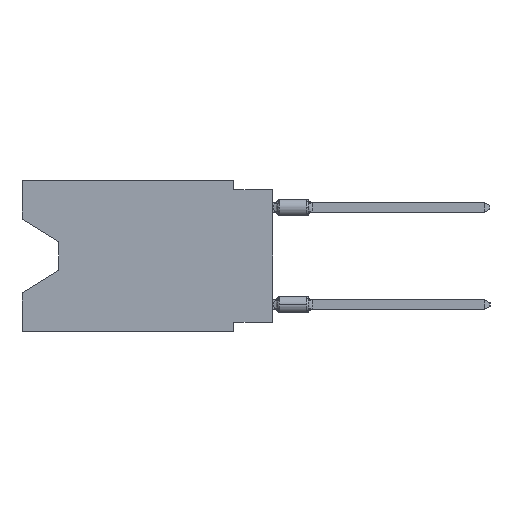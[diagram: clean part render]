
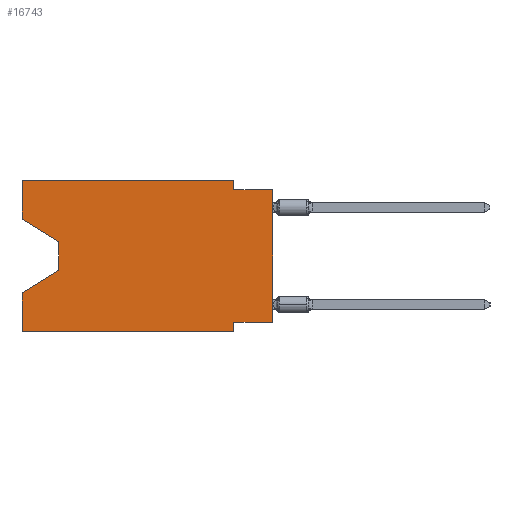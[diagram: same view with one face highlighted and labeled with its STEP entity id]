
A CAD part, left-side view. The second image highlights one B-rep face of the part: STEP entity #16743.
In plain terms, the highlighted planar face has unit normal (-1, 0, 0).
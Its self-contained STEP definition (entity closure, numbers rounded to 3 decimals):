
#596 = CARTESIAN_POINT ( 'NONE',  ( 0., 13.97, -4.013 ) ) ;
#653 = LINE ( 'NONE', #23983, #19637 ) ;
#842 = LINE ( 'NONE', #13902, #12736 ) ;
#1052 = ORIENTED_EDGE ( 'NONE', *, *, #29931, .T. ) ;
#1077 = CARTESIAN_POINT ( 'NONE',  ( 0., 2.54, -9.906 ) ) ;
#1109 = LINE ( 'NONE', #29670, #18030 ) ;
#2143 = FACE_OUTER_BOUND ( 'NONE', #13013, .T. ) ;
#2547 = DIRECTION ( 'NONE',  ( 0., -1., 0. ) ) ;
#2576 = ORIENTED_EDGE ( 'NONE', *, *, #39382, .F. ) ;
#3517 = VECTOR ( 'NONE', #20984, 1000. ) ;
#3656 = CARTESIAN_POINT ( 'NONE',  ( 0., 0., -0.635 ) ) ;
#4217 = LINE ( 'NONE', #11286, #37618 ) ;
#4833 = CARTESIAN_POINT ( 'NONE',  ( 0., 16.383, -2.546 ) ) ;
#5164 = ORIENTED_EDGE ( 'NONE', *, *, #32402, .F. ) ;
#5377 = DIRECTION ( 'NONE',  ( 0., 0., -1. ) ) ;
#6178 = VERTEX_POINT ( 'NONE', #6815 ) ;
#6801 = VERTEX_POINT ( 'NONE', #10830 ) ;
#6815 = CARTESIAN_POINT ( 'NONE',  ( 0., 2.54, -0.635 ) ) ;
#7236 = CARTESIAN_POINT ( 'NONE',  ( 0., 0., -0.635 ) ) ;
#7422 = DIRECTION ( 'NONE',  ( 0., 0., -1. ) ) ;
#7446 = VECTOR ( 'NONE', #29320, 1000. ) ;
#7562 = DIRECTION ( 'NONE',  ( 1., 0., 0. ) ) ;
#7871 = DIRECTION ( 'NONE',  ( 0., -1., 0. ) ) ;
#8173 = VERTEX_POINT ( 'NONE', #15523 ) ;
#10216 = ORIENTED_EDGE ( 'NONE', *, *, #24145, .F. ) ;
#10549 = CARTESIAN_POINT ( 'NONE',  ( 0., 2.54, 0. ) ) ;
#10830 = CARTESIAN_POINT ( 'NONE',  ( 0., 16.383, 0. ) ) ;
#11286 = CARTESIAN_POINT ( 'NONE',  ( 0., 16.383, 0. ) ) ;
#12124 = VECTOR ( 'NONE', #7871, 1000. ) ;
#12736 = VECTOR ( 'NONE', #7422, 1000. ) ;
#13013 = EDGE_LOOP ( 'NONE', ( #22837, #1052, #39787, #10216, #38677, #34655, #5164, #20052, #34958, #22917, #28257, #2576 ) ) ;
#13902 = CARTESIAN_POINT ( 'NONE',  ( 0., 13.97, -4.013 ) ) ;
#13945 = EDGE_CURVE ( 'NONE', #6801, #41479, #1109, .T. ) ;
#14997 = VECTOR ( 'NONE', #21978, 1000. ) ;
#15391 = CARTESIAN_POINT ( 'NONE',  ( 0., 16.383, -9.906 ) ) ;
#15523 = CARTESIAN_POINT ( 'NONE',  ( 0., 2.54, -9.271 ) ) ;
#15562 = LINE ( 'NONE', #31651, #14997 ) ;
#16112 = VECTOR ( 'NONE', #40861, 1000. ) ;
#16743 = ADVANCED_FACE ( 'NONE', ( #2143 ), #23850, .F. ) ;
#16860 = CARTESIAN_POINT ( 'NONE',  ( 0., 13.97, -5.893 ) ) ;
#18030 = VECTOR ( 'NONE', #22798, 1000. ) ;
#18427 = EDGE_CURVE ( 'NONE', #8173, #28318, #37100, .T. ) ;
#19011 = VECTOR ( 'NONE', #2547, 1000. ) ;
#19637 = VECTOR ( 'NONE', #39692, 1000. ) ;
#19661 = LINE ( 'NONE', #16860, #7446 ) ;
#20052 = ORIENTED_EDGE ( 'NONE', *, *, #29200, .T. ) ;
#20984 = DIRECTION ( 'NONE',  ( 0., 0., -1. ) ) ;
#21365 = CARTESIAN_POINT ( 'NONE',  ( 0., 13.97, -5.893 ) ) ;
#21547 = CARTESIAN_POINT ( 'NONE',  ( 0., 16.383, -9.906 ) ) ;
#21718 = CARTESIAN_POINT ( 'NONE',  ( 0., 16.383, -2.546 ) ) ;
#21978 = DIRECTION ( 'NONE',  ( 0., 0., -1. ) ) ;
#22300 = VERTEX_POINT ( 'NONE', #21547 ) ;
#22470 = LINE ( 'NONE', #32545, #40842 ) ;
#22726 = EDGE_CURVE ( 'NONE', #41015, #39270, #27740, .T. ) ;
#22798 = DIRECTION ( 'NONE',  ( 0., -1., 0. ) ) ;
#22837 = ORIENTED_EDGE ( 'NONE', *, *, #22726, .T. ) ;
#22917 = ORIENTED_EDGE ( 'NONE', *, *, #39469, .F. ) ;
#22973 = CARTESIAN_POINT ( 'NONE',  ( 0., 2.54, -9.906 ) ) ;
#23195 = CARTESIAN_POINT ( 'NONE',  ( 0., 16.383, 0. ) ) ;
#23850 = PLANE ( 'NONE',  #33568 ) ;
#23983 = CARTESIAN_POINT ( 'NONE',  ( 0., 0., -9.271 ) ) ;
#24145 = EDGE_CURVE ( 'NONE', #22300, #27366, #36305, .T. ) ;
#24353 = DIRECTION ( 'NONE',  ( 0., 0., 1. ) ) ;
#26185 = EDGE_CURVE ( 'NONE', #37577, #27366, #19661, .T. ) ;
#26486 = VECTOR ( 'NONE', #30275, 1000. ) ;
#27182 = LINE ( 'NONE', #7236, #12124 ) ;
#27366 = VERTEX_POINT ( 'NONE', #38624 ) ;
#27740 = LINE ( 'NONE', #21718, #16112 ) ;
#28257 = ORIENTED_EDGE ( 'NONE', *, *, #13945, .F. ) ;
#28318 = VERTEX_POINT ( 'NONE', #22973 ) ;
#29200 = EDGE_CURVE ( 'NONE', #40311, #36917, #22470, .T. ) ;
#29320 = DIRECTION ( 'NONE',  ( 0., 0.855, -0.519 ) ) ;
#29531 = DIRECTION ( 'NONE',  ( 0., 0., 1. ) ) ;
#29670 = CARTESIAN_POINT ( 'NONE',  ( 0., 16.383, 0. ) ) ;
#29931 = EDGE_CURVE ( 'NONE', #39270, #37577, #842, .T. ) ;
#30275 = DIRECTION ( 'NONE',  ( 0., 0., 1. ) ) ;
#31578 = EDGE_CURVE ( 'NONE', #22300, #28318, #41598, .T. ) ;
#31651 = CARTESIAN_POINT ( 'NONE',  ( 0., 2.54, 0. ) ) ;
#32402 = EDGE_CURVE ( 'NONE', #40311, #8173, #653, .T. ) ;
#32545 = CARTESIAN_POINT ( 'NONE',  ( 0., 0., 0. ) ) ;
#33568 = AXIS2_PLACEMENT_3D ( 'NONE', #34740, #7562, #5377 ) ;
#34086 = CARTESIAN_POINT ( 'NONE',  ( 0., 0., -9.271 ) ) ;
#34655 = ORIENTED_EDGE ( 'NONE', *, *, #18427, .F. ) ;
#34740 = CARTESIAN_POINT ( 'NONE',  ( 0., 16.383, 0. ) ) ;
#34958 = ORIENTED_EDGE ( 'NONE', *, *, #37454, .F. ) ;
#36305 = LINE ( 'NONE', #23195, #26486 ) ;
#36917 = VERTEX_POINT ( 'NONE', #3656 ) ;
#37100 = LINE ( 'NONE', #1077, #3517 ) ;
#37454 = EDGE_CURVE ( 'NONE', #6178, #36917, #27182, .T. ) ;
#37577 = VERTEX_POINT ( 'NONE', #21365 ) ;
#37618 = VECTOR ( 'NONE', #24353, 1000. ) ;
#38624 = CARTESIAN_POINT ( 'NONE',  ( 0., 16.383, -7.36 ) ) ;
#38677 = ORIENTED_EDGE ( 'NONE', *, *, #31578, .T. ) ;
#39270 = VERTEX_POINT ( 'NONE', #596 ) ;
#39382 = EDGE_CURVE ( 'NONE', #41015, #6801, #4217, .T. ) ;
#39469 = EDGE_CURVE ( 'NONE', #41479, #6178, #15562, .T. ) ;
#39692 = DIRECTION ( 'NONE',  ( 0., 1., 0. ) ) ;
#39787 = ORIENTED_EDGE ( 'NONE', *, *, #26185, .T. ) ;
#40311 = VERTEX_POINT ( 'NONE', #34086 ) ;
#40842 = VECTOR ( 'NONE', #29531, 1000. ) ;
#40861 = DIRECTION ( 'NONE',  ( 0., -0.855, -0.519 ) ) ;
#41015 = VERTEX_POINT ( 'NONE', #4833 ) ;
#41479 = VERTEX_POINT ( 'NONE', #10549 ) ;
#41598 = LINE ( 'NONE', #15391, #19011 ) ;
